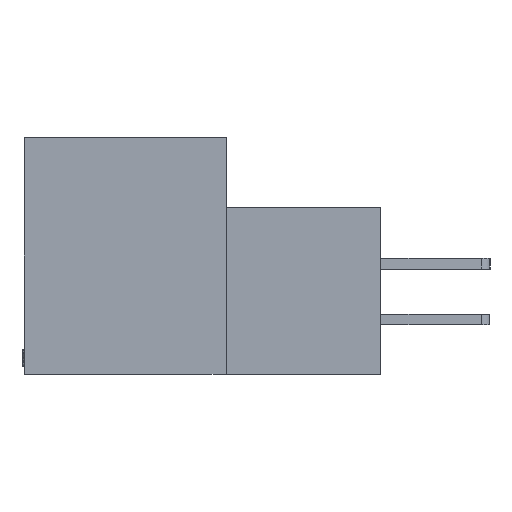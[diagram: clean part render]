
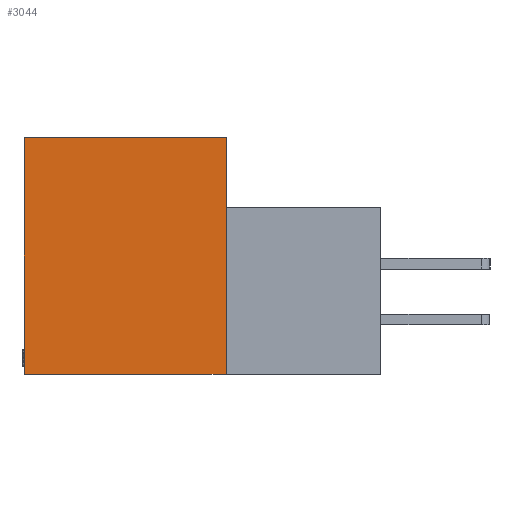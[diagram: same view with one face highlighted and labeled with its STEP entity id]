
A CAD part, left-side view. The second image highlights one B-rep face of the part: STEP entity #3044.
In plain terms, the highlighted planar face has unit normal (-1, 0, 0).
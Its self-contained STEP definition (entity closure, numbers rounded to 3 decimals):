
#1261 = EDGE_CURVE ( 'NONE', #10951, #1968, #4066, .T. ) ;
#1968 = VERTEX_POINT ( 'NONE', #10770 ) ;
#3044 = ADVANCED_FACE ( 'NONE', ( #6314 ), #22184, .F. ) ;
#3393 = ORIENTED_EDGE ( 'NONE', *, *, #1261, .F. ) ;
#4066 = LINE ( 'NONE', #14285, #9877 ) ;
#4254 = EDGE_CURVE ( 'NONE', #23476, #10951, #15815, .T. ) ;
#4610 = LINE ( 'NONE', #21329, #20571 ) ;
#5480 = EDGE_LOOP ( 'NONE', ( #11778, #3393, #11618, #17905 ) ) ;
#5587 = DIRECTION ( 'NONE',  ( 0., 0., -1. ) ) ;
#6314 = FACE_OUTER_BOUND ( 'NONE', #5480, .T. ) ;
#6521 = DIRECTION ( 'NONE',  ( 0., 1., 0. ) ) ;
#6652 = DIRECTION ( 'NONE',  ( 0., 0., 1. ) ) ;
#8560 = DIRECTION ( 'NONE',  ( 0., -1., 0. ) ) ;
#9877 = VECTOR ( 'NONE', #12502, 1000. ) ;
#10027 = VECTOR ( 'NONE', #6521, 1000. ) ;
#10763 = EDGE_CURVE ( 'NONE', #1968, #20815, #22761, .T. ) ;
#10770 = CARTESIAN_POINT ( 'NONE',  ( 0., 0., -13.487 ) ) ;
#10951 = VERTEX_POINT ( 'NONE', #21774 ) ;
#11089 = DIRECTION ( 'NONE',  ( 1., 0., 0. ) ) ;
#11618 = ORIENTED_EDGE ( 'NONE', *, *, #4254, .F. ) ;
#11778 = ORIENTED_EDGE ( 'NONE', *, *, #10763, .F. ) ;
#12502 = DIRECTION ( 'NONE',  ( 0., 0., -1. ) ) ;
#12884 = CARTESIAN_POINT ( 'NONE',  ( 0., 11.506, -13.487 ) ) ;
#13102 = CARTESIAN_POINT ( 'NONE',  ( 0., 11.506, 0. ) ) ;
#13208 = VECTOR ( 'NONE', #8560, 1000. ) ;
#14285 = CARTESIAN_POINT ( 'NONE',  ( 0., 0., 0. ) ) ;
#15212 = AXIS2_PLACEMENT_3D ( 'NONE', #16641, #11089, #5587 ) ;
#15815 = LINE ( 'NONE', #16173, #13208 ) ;
#15922 = CARTESIAN_POINT ( 'NONE',  ( 0., -8.814, -13.487 ) ) ;
#16173 = CARTESIAN_POINT ( 'NONE',  ( 0., 11.506, 0. ) ) ;
#16641 = CARTESIAN_POINT ( 'NONE',  ( 0., 0., 0. ) ) ;
#17905 = ORIENTED_EDGE ( 'NONE', *, *, #21021, .F. ) ;
#20571 = VECTOR ( 'NONE', #6652, 1000. ) ;
#20815 = VERTEX_POINT ( 'NONE', #12884 ) ;
#21021 = EDGE_CURVE ( 'NONE', #20815, #23476, #4610, .T. ) ;
#21329 = CARTESIAN_POINT ( 'NONE',  ( 0., 11.506, -13.487 ) ) ;
#21774 = CARTESIAN_POINT ( 'NONE',  ( 0., 0., 0. ) ) ;
#22184 = PLANE ( 'NONE',  #15212 ) ;
#22761 = LINE ( 'NONE', #15922, #10027 ) ;
#23476 = VERTEX_POINT ( 'NONE', #13102 ) ;
